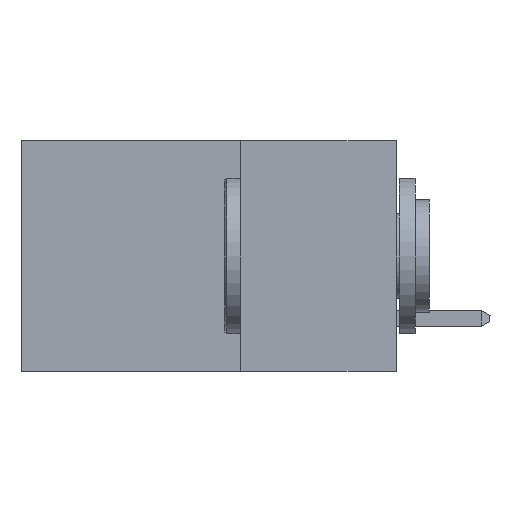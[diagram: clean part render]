
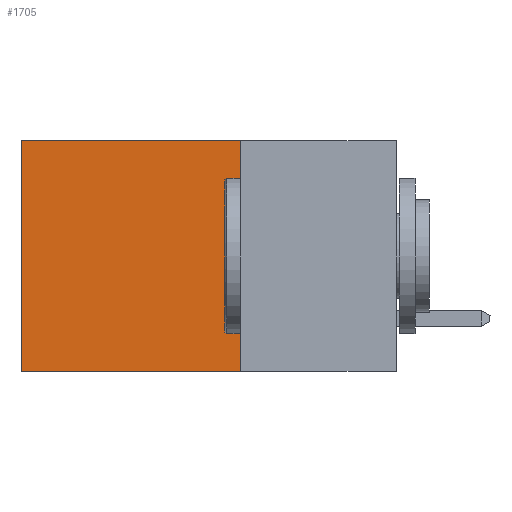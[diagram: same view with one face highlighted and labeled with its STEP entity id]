
A CAD part, left-side view. The second image highlights one B-rep face of the part: STEP entity #1705.
In plain terms, the highlighted planar face has unit normal (-1, 0, 0).
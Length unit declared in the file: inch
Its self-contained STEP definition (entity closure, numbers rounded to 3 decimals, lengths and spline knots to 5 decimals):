
#597 = EDGE_CURVE ( 'NONE', #13231, #7018, #4297, .T. ) ;
#1475 = VERTEX_POINT ( 'NONE', #6576 ) ;
#1494 = LINE ( 'NONE', #3039, #5239 ) ;
#1560 = ORIENTED_EDGE ( 'NONE', *, *, #1646, .F. ) ;
#1646 = EDGE_CURVE ( 'NONE', #1475, #7018, #11475, .T. ) ;
#1705 = ADVANCED_FACE ( 'NONE', ( #4061 ), #15532, .F. ) ;
#1991 = VECTOR ( 'NONE', #14140, 39.37008 ) ;
#2344 = DIRECTION ( 'NONE',  ( 1., 0., 0. ) ) ;
#2349 = DIRECTION ( 'NONE',  ( 0., 0., -1. ) ) ;
#2802 = CARTESIAN_POINT ( 'NONE',  ( 0.2615, 0.25, -0.37 ) ) ;
#3039 = CARTESIAN_POINT ( 'NONE',  ( 0.2615, 0.25, -0.37 ) ) ;
#3280 = CARTESIAN_POINT ( 'NONE',  ( 0.2615, 0.25, -0.37 ) ) ;
#3585 = CARTESIAN_POINT ( 'NONE',  ( 0.2615, 0.6, 0. ) ) ;
#3765 = DIRECTION ( 'NONE',  ( 0., 1., 0. ) ) ;
#4061 = FACE_OUTER_BOUND ( 'NONE', #10564, .T. ) ;
#4297 = LINE ( 'NONE', #5184, #5123 ) ;
#5123 = VECTOR ( 'NONE', #12034, 39.37008 ) ;
#5184 = CARTESIAN_POINT ( 'NONE',  ( 0.2615, 0.6, -0.37 ) ) ;
#5239 = VECTOR ( 'NONE', #11749, 39.37008 ) ;
#5706 = CARTESIAN_POINT ( 'NONE',  ( 0.2615, 0.25, 0. ) ) ;
#6332 = CARTESIAN_POINT ( 'NONE',  ( 0.2615, 0.6, -0.37 ) ) ;
#6576 = CARTESIAN_POINT ( 'NONE',  ( 0.2615, 0.25, -0.37 ) ) ;
#7018 = VERTEX_POINT ( 'NONE', #6332 ) ;
#7075 = VERTEX_POINT ( 'NONE', #5706 ) ;
#7437 = ORIENTED_EDGE ( 'NONE', *, *, #8182, .T. ) ;
#8136 = ORIENTED_EDGE ( 'NONE', *, *, #14058, .F. ) ;
#8182 = EDGE_CURVE ( 'NONE', #7075, #13231, #8737, .T. ) ;
#8737 = LINE ( 'NONE', #14092, #1991 ) ;
#10564 = EDGE_LOOP ( 'NONE', ( #13795, #1560, #8136, #7437 ) ) ;
#11475 = LINE ( 'NONE', #3280, #14572 ) ;
#11749 = DIRECTION ( 'NONE',  ( 0., 0., -1. ) ) ;
#12034 = DIRECTION ( 'NONE',  ( 0., 0., -1. ) ) ;
#12406 = AXIS2_PLACEMENT_3D ( 'NONE', #2802, #2344, #2349 ) ;
#13231 = VERTEX_POINT ( 'NONE', #3585 ) ;
#13795 = ORIENTED_EDGE ( 'NONE', *, *, #597, .T. ) ;
#14058 = EDGE_CURVE ( 'NONE', #7075, #1475, #1494, .T. ) ;
#14092 = CARTESIAN_POINT ( 'NONE',  ( 0.2615, 0.25, 0. ) ) ;
#14140 = DIRECTION ( 'NONE',  ( 0., 1., 0. ) ) ;
#14572 = VECTOR ( 'NONE', #3765, 39.37008 ) ;
#15532 = PLANE ( 'NONE',  #12406 ) ;
